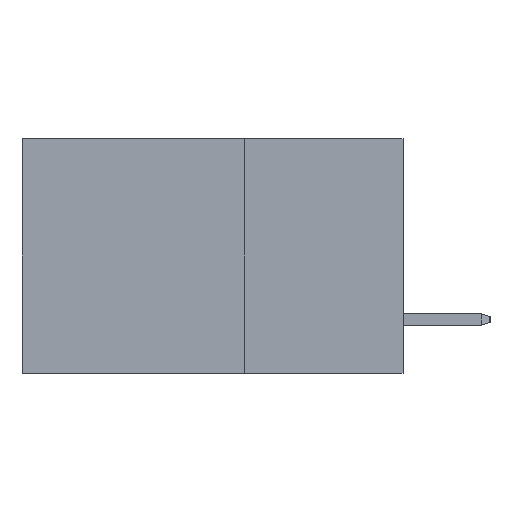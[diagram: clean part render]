
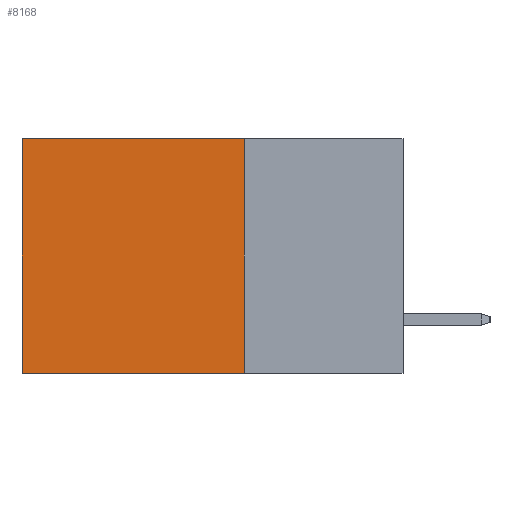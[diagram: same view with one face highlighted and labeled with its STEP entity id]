
A CAD part, left-side view. The second image highlights one B-rep face of the part: STEP entity #8168.
In plain terms, the highlighted planar face has unit normal (-1, 0, 0).
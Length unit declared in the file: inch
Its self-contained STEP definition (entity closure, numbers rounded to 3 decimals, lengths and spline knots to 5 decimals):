
#58 = CARTESIAN_POINT ( 'NONE',  ( 0.2875, 0.25, -0.37 ) ) ;
#810 = CARTESIAN_POINT ( 'NONE',  ( 0.2875, 0.6, 0. ) ) ;
#1117 = LINE ( 'NONE', #6896, #6180 ) ;
#1230 = CARTESIAN_POINT ( 'NONE',  ( 0.2875, 0.25, 0. ) ) ;
#1552 = EDGE_CURVE ( 'NONE', #14060, #13237, #17466, .T. ) ;
#1765 = ORIENTED_EDGE ( 'NONE', *, *, #7544, .T. ) ;
#2290 = DIRECTION ( 'NONE',  ( 0., 0., -1. ) ) ;
#2412 = VECTOR ( 'NONE', #2290, 39.37008 ) ;
#2609 = PLANE ( 'NONE',  #9599 ) ;
#3027 = CARTESIAN_POINT ( 'NONE',  ( 0.2875, 0.6, -0.37 ) ) ;
#4929 = CARTESIAN_POINT ( 'NONE',  ( 0.2875, 0.25, -0.37 ) ) ;
#5944 = ORIENTED_EDGE ( 'NONE', *, *, #1552, .F. ) ;
#6180 = VECTOR ( 'NONE', #6803, 39.37008 ) ;
#6803 = DIRECTION ( 'NONE',  ( 0., 1., 0. ) ) ;
#6848 = EDGE_CURVE ( 'NONE', #11876, #14531, #1117, .T. ) ;
#6896 = CARTESIAN_POINT ( 'NONE',  ( 0.2875, 0.25, 0. ) ) ;
#7544 = EDGE_CURVE ( 'NONE', #14531, #13237, #13437, .T. ) ;
#8168 = ADVANCED_FACE ( 'NONE', ( #9533 ), #2609, .F. ) ;
#8181 = DIRECTION ( 'NONE',  ( 1., 0., 0. ) ) ;
#9307 = VECTOR ( 'NONE', #11004, 39.37008 ) ;
#9352 = LINE ( 'NONE', #14944, #9307 ) ;
#9533 = FACE_OUTER_BOUND ( 'NONE', #11044, .T. ) ;
#9599 = AXIS2_PLACEMENT_3D ( 'NONE', #1230, #8181, #11100 ) ;
#10488 = DIRECTION ( 'NONE',  ( 0., 1., 0. ) ) ;
#11004 = DIRECTION ( 'NONE',  ( 0., 0., -1. ) ) ;
#11044 = EDGE_LOOP ( 'NONE', ( #1765, #5944, #12848, #11274 ) ) ;
#11100 = DIRECTION ( 'NONE',  ( 0., 0., -1. ) ) ;
#11274 = ORIENTED_EDGE ( 'NONE', *, *, #6848, .T. ) ;
#11623 = VECTOR ( 'NONE', #10488, 39.37008 ) ;
#11831 = EDGE_CURVE ( 'NONE', #11876, #14060, #9352, .T. ) ;
#11876 = VERTEX_POINT ( 'NONE', #14194 ) ;
#12848 = ORIENTED_EDGE ( 'NONE', *, *, #11831, .F. ) ;
#13237 = VERTEX_POINT ( 'NONE', #3027 ) ;
#13437 = LINE ( 'NONE', #810, #2412 ) ;
#14060 = VERTEX_POINT ( 'NONE', #58 ) ;
#14194 = CARTESIAN_POINT ( 'NONE',  ( 0.2875, 0.25, 0. ) ) ;
#14531 = VERTEX_POINT ( 'NONE', #16870 ) ;
#14944 = CARTESIAN_POINT ( 'NONE',  ( 0.2875, 0.25, 0. ) ) ;
#16870 = CARTESIAN_POINT ( 'NONE',  ( 0.2875, 0.6, 0. ) ) ;
#17466 = LINE ( 'NONE', #4929, #11623 ) ;
